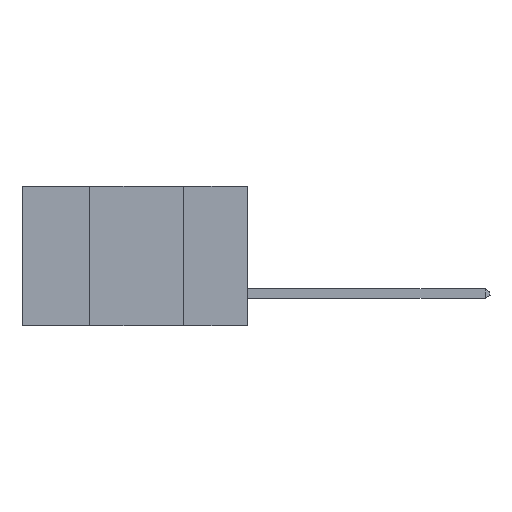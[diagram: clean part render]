
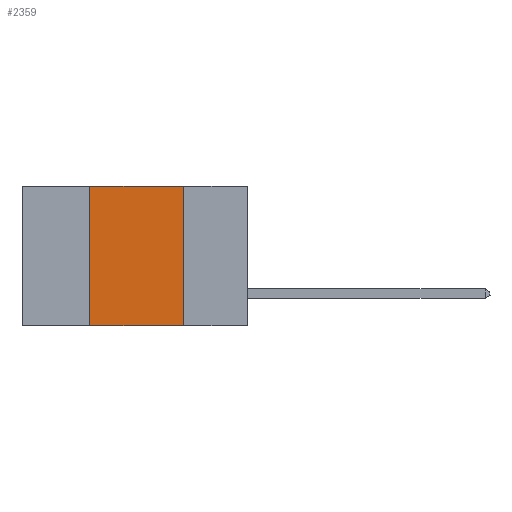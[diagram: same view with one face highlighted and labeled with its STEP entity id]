
A CAD part, left-side view. The second image highlights one B-rep face of the part: STEP entity #2359.
In plain terms, the highlighted planar face has unit normal (-1, 0, 0).
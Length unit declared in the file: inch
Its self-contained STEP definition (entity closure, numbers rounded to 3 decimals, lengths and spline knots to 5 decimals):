
#216 = LINE ( 'NONE', #6080, #9608 ) ;
#1374 = VERTEX_POINT ( 'NONE', #4811 ) ;
#1660 = EDGE_CURVE ( 'NONE', #5811, #1374, #6668, .T. ) ;
#2063 = ORIENTED_EDGE ( 'NONE', *, *, #1660, .F. ) ;
#2359 = ADVANCED_FACE ( 'NONE', ( #5090 ), #3330, .F. ) ;
#2509 = CARTESIAN_POINT ( 'NONE',  ( 0., 0.17, -0.37 ) ) ;
#2898 = DIRECTION ( 'NONE',  ( 0., -1., 0. ) ) ;
#3330 = PLANE ( 'NONE',  #12223 ) ;
#4319 = EDGE_CURVE ( 'NONE', #9544, #5811, #9050, .T. ) ;
#4811 = CARTESIAN_POINT ( 'NONE',  ( 0., 0.17, 0. ) ) ;
#5090 = FACE_OUTER_BOUND ( 'NONE', #12739, .T. ) ;
#5188 = ORIENTED_EDGE ( 'NONE', *, *, #7839, .T. ) ;
#5370 = DIRECTION ( 'NONE',  ( 1., 0., 0. ) ) ;
#5811 = VERTEX_POINT ( 'NONE', #8619 ) ;
#5873 = VECTOR ( 'NONE', #2898, 39.37008 ) ;
#6080 = CARTESIAN_POINT ( 'NONE',  ( 0., 0.17, 0. ) ) ;
#6145 = EDGE_CURVE ( 'NONE', #1374, #9387, #216, .T. ) ;
#6668 = LINE ( 'NONE', #10653, #9575 ) ;
#6782 = DIRECTION ( 'NONE',  ( 0., -1., 0. ) ) ;
#6976 = CARTESIAN_POINT ( 'NONE',  ( 0., 0.42, -0.37 ) ) ;
#7839 = EDGE_CURVE ( 'NONE', #9544, #9387, #8491, .T. ) ;
#8491 = LINE ( 'NONE', #11072, #5873 ) ;
#8619 = CARTESIAN_POINT ( 'NONE',  ( 0., 0.42, 0. ) ) ;
#9044 = DIRECTION ( 'NONE',  ( 0., 0., -1. ) ) ;
#9050 = LINE ( 'NONE', #10310, #9978 ) ;
#9357 = DIRECTION ( 'NONE',  ( 0., 0., 1. ) ) ;
#9387 = VERTEX_POINT ( 'NONE', #2509 ) ;
#9544 = VERTEX_POINT ( 'NONE', #6976 ) ;
#9575 = VECTOR ( 'NONE', #6782, 39.37008 ) ;
#9608 = VECTOR ( 'NONE', #9044, 39.37008 ) ;
#9672 = ORIENTED_EDGE ( 'NONE', *, *, #4319, .F. ) ;
#9978 = VECTOR ( 'NONE', #9357, 39.37008 ) ;
#10279 = CARTESIAN_POINT ( 'NONE',  ( 0., 0.6, 0. ) ) ;
#10310 = CARTESIAN_POINT ( 'NONE',  ( 0., 0.42, 0. ) ) ;
#10480 = ORIENTED_EDGE ( 'NONE', *, *, #6145, .F. ) ;
#10653 = CARTESIAN_POINT ( 'NONE',  ( 0., 0.6, 0. ) ) ;
#11072 = CARTESIAN_POINT ( 'NONE',  ( 0., 0.6, -0.37 ) ) ;
#12223 = AXIS2_PLACEMENT_3D ( 'NONE', #10279, #5370, #12317 ) ;
#12317 = DIRECTION ( 'NONE',  ( 0., 0., -1. ) ) ;
#12739 = EDGE_LOOP ( 'NONE', ( #10480, #2063, #9672, #5188 ) ) ;
